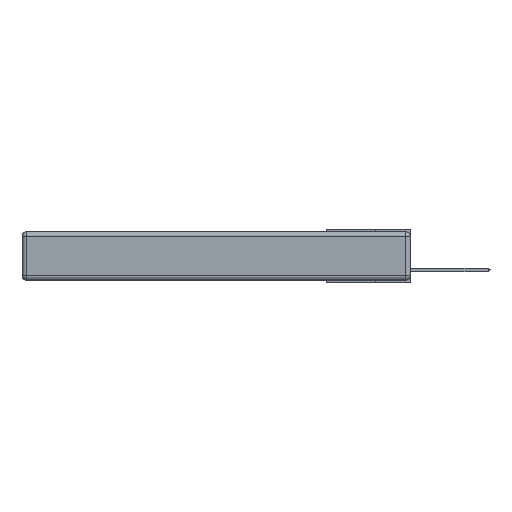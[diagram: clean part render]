
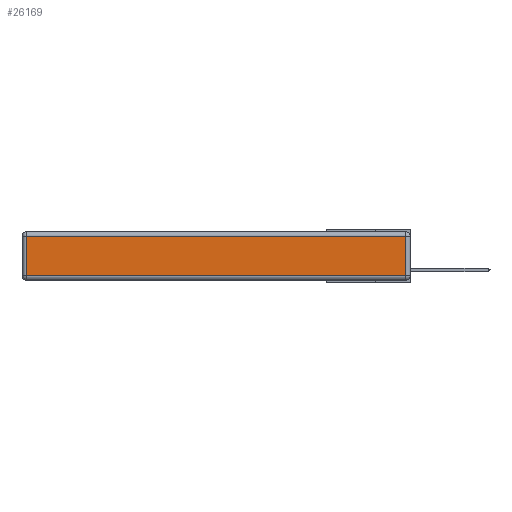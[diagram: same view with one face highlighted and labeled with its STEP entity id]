
A CAD part, left-side view. The second image highlights one B-rep face of the part: STEP entity #26169.
In plain terms, the highlighted planar face has unit normal (-1, 0, 0).
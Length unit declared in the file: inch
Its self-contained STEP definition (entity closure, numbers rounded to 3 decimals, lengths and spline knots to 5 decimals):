
#1364 = CARTESIAN_POINT ( 'NONE',  ( 0., 2.72, -0.03 ) ) ;
#1944 = CARTESIAN_POINT ( 'NONE',  ( 0., 0.03, -0.343 ) ) ;
#2122 = ORIENTED_EDGE ( 'NONE', *, *, #25444, .T. ) ;
#2416 = CARTESIAN_POINT ( 'NONE',  ( 0., 2.75, -0.03 ) ) ;
#2453 = CARTESIAN_POINT ( 'NONE',  ( 0., 0., -0.343 ) ) ;
#2907 = VECTOR ( 'NONE', #22818, 39.37008 ) ;
#3293 = VECTOR ( 'NONE', #7055, 39.37008 ) ;
#6330 = EDGE_CURVE ( 'NONE', #8305, #22594, #21017, .T. ) ;
#7055 = DIRECTION ( 'NONE',  ( 0., -1., 0. ) ) ;
#7876 = ORIENTED_EDGE ( 'NONE', *, *, #6330, .T. ) ;
#7943 = DIRECTION ( 'NONE',  ( 0., 0., 1. ) ) ;
#8305 = VERTEX_POINT ( 'NONE', #23126 ) ;
#8427 = DIRECTION ( 'NONE',  ( 0., 0., 1. ) ) ;
#8743 = VECTOR ( 'NONE', #7943, 39.37008 ) ;
#8983 = FACE_OUTER_BOUND ( 'NONE', #16215, .T. ) ;
#10400 = PLANE ( 'NONE',  #11731 ) ;
#11731 = AXIS2_PLACEMENT_3D ( 'NONE', #2453, #18913, #8427 ) ;
#12711 = EDGE_CURVE ( 'NONE', #22594, #17381, #18686, .T. ) ;
#13036 = VECTOR ( 'NONE', #16803, 39.37008 ) ;
#14990 = VERTEX_POINT ( 'NONE', #25499 ) ;
#16215 = EDGE_LOOP ( 'NONE', ( #2122, #7876, #20280, #24750 ) ) ;
#16803 = DIRECTION ( 'NONE',  ( 0., 0., -1. ) ) ;
#17325 = CARTESIAN_POINT ( 'NONE',  ( 0., 0., -0.313 ) ) ;
#17381 = VERTEX_POINT ( 'NONE', #1364 ) ;
#17880 = LINE ( 'NONE', #23087, #13036 ) ;
#18686 = LINE ( 'NONE', #2416, #2907 ) ;
#18913 = DIRECTION ( 'NONE',  ( -1., 0., 0. ) ) ;
#20013 = LINE ( 'NONE', #17325, #3293 ) ;
#20280 = ORIENTED_EDGE ( 'NONE', *, *, #12711, .T. ) ;
#21017 = LINE ( 'NONE', #1944, #8743 ) ;
#21408 = CARTESIAN_POINT ( 'NONE',  ( 0., 0.03, -0.03 ) ) ;
#22594 = VERTEX_POINT ( 'NONE', #21408 ) ;
#22818 = DIRECTION ( 'NONE',  ( 0., 1., 0. ) ) ;
#23087 = CARTESIAN_POINT ( 'NONE',  ( 0., 2.72, -0.343 ) ) ;
#23103 = EDGE_CURVE ( 'NONE', #17381, #14990, #17880, .T. ) ;
#23126 = CARTESIAN_POINT ( 'NONE',  ( 0., 0.03, -0.313 ) ) ;
#24750 = ORIENTED_EDGE ( 'NONE', *, *, #23103, .T. ) ;
#25444 = EDGE_CURVE ( 'NONE', #14990, #8305, #20013, .T. ) ;
#25499 = CARTESIAN_POINT ( 'NONE',  ( 0., 2.72, -0.313 ) ) ;
#26169 = ADVANCED_FACE ( 'NONE', ( #8983 ), #10400, .T. ) ;
